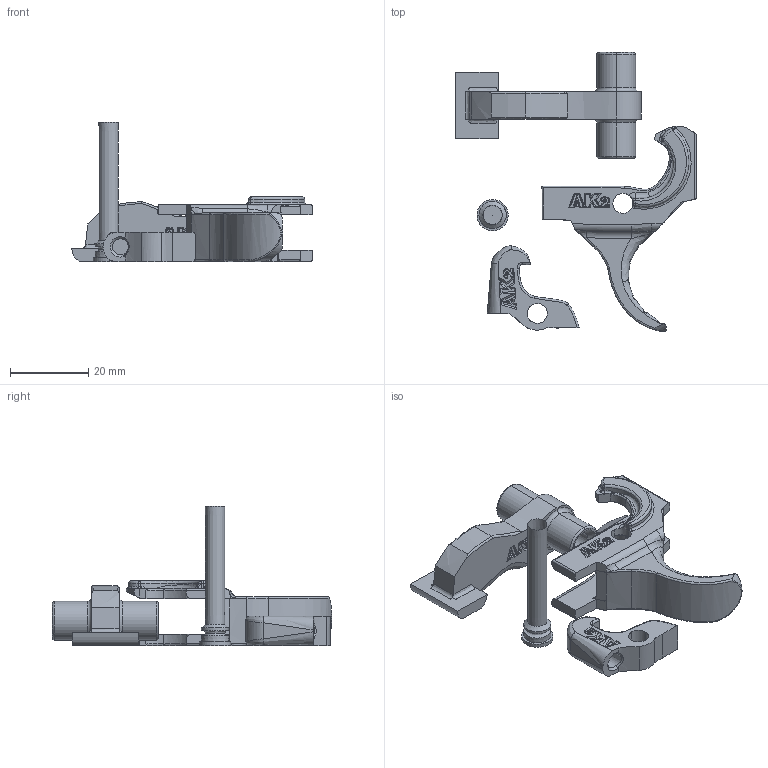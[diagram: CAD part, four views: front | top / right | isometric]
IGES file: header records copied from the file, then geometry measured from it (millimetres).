
Global section: file name: No Iges File Name specified; native system: Autodesk Inventor 2012; preprocessor: AutoDesk Inventor Iges Exporter R2012; author: ohammer; date: 20121007.023921; units: millimetre
Bounding box: 61.5 x 71.24 x 35.58 mm (x, y, z)
Volume: 12556.1 mm3; surface area: 8966.5 mm2
Topology: 4 solids, 4 shells, 503 faces, 1371 edges, 940 vertices
Faces by surface type: plane 245, bspline 194, revolution 23, cylinder 23, cone 7, torus 7, sphere 4
